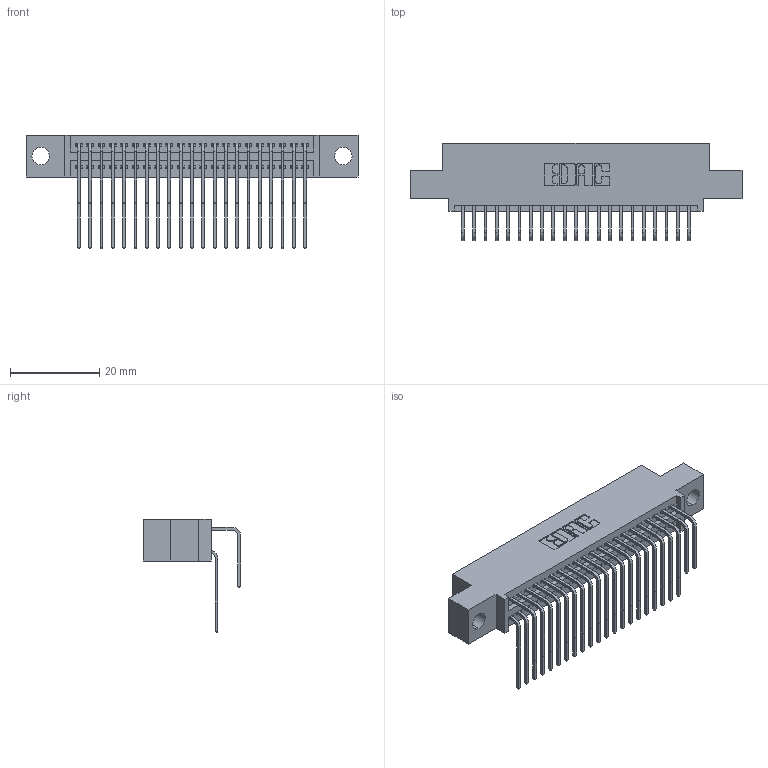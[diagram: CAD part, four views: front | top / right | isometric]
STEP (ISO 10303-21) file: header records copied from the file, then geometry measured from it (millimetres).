
FILE_DESCRIPTION (( 'STEP AP203' ), '1' );
FILE_NAME ('395-042-558-504.STEP', '2021-06-16T22:25:17', ( '' ), ( '' ), 'SwSTEP 2.0', 'SolidWorks 2020', '' );
FILE_SCHEMA (( 'CONFIG_CONTROL_DESIGN' ));
Length unit declared in the file: inch
Products named in the file (4): 345 Part_0.110 Offset - 0.156 Dia-TI; 345-292-001_558 559 Tail - 1; 345-292-001_558 Tail - 2; 395-042-558-504
Assembly tree (43 placements, depth 2):
  395-042-558-504
    345 Part_0.110 Offset - 0.156 Dia-TI
    345-292-001_558 559 Tail - 1  x21
    345-292-001_558 Tail - 2  x21
Bounding box: 74.55 x 21.83 x 25.53 mm (x, y, z)
Volume: 7109.8 mm3; surface area: 11186.5 mm2
Topology: 43 solids, 43 shells, 2328 faces, 6899 edges, 4542 vertices
Faces by surface type: plane 1568, cylinder 760
Entity records: 21507 total; most frequent: CARTESIAN_POINT 3677, ORIENTED_EDGE 3558, DIRECTION 3239, EDGE_CURVE 1779, LINE 1523, VECTOR 1523, VERTEX_POINT 1182, AXIS2_PLACEMENT_3D 858
